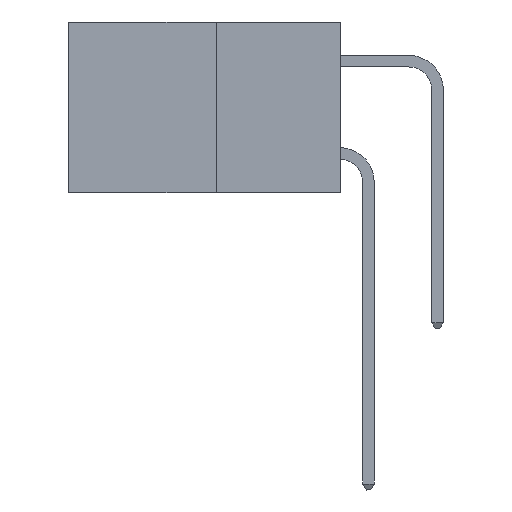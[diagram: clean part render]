
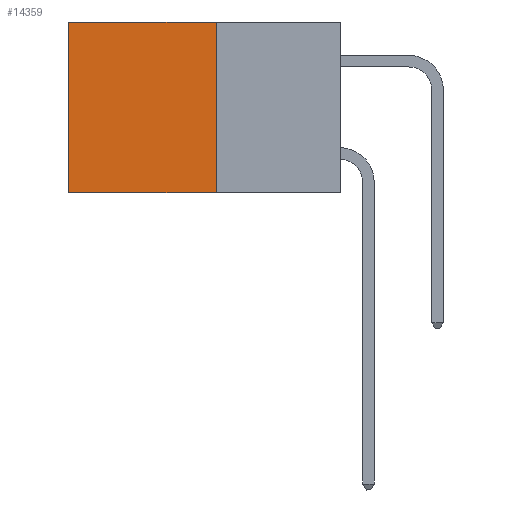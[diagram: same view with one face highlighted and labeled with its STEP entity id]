
A CAD part, left-side view. The second image highlights one B-rep face of the part: STEP entity #14359.
In plain terms, the highlighted planar face has unit normal (-1, 0, 0).
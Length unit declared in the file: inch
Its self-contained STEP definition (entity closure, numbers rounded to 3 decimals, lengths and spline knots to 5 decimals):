
#228 = VECTOR ( 'NONE', #15849, 39.37008 ) ;
#976 = DIRECTION ( 'NONE',  ( 0., 0., -1. ) ) ;
#2099 = VECTOR ( 'NONE', #976, 39.37008 ) ;
#2131 = FACE_OUTER_BOUND ( 'NONE', #4320, .T. ) ;
#3028 = VERTEX_POINT ( 'NONE', #15175 ) ;
#4080 = DIRECTION ( 'NONE',  ( 1., 0., 0. ) ) ;
#4320 = EDGE_LOOP ( 'NONE', ( #19175, #17777, #12674, #13110 ) ) ;
#4397 = CARTESIAN_POINT ( 'NONE',  ( 0.277, 0.59, -0.37 ) ) ;
#5639 = LINE ( 'NONE', #15153, #228 ) ;
#6575 = EDGE_CURVE ( 'NONE', #3028, #13908, #5639, .T. ) ;
#7083 = AXIS2_PLACEMENT_3D ( 'NONE', #14992, #4080, #16765 ) ;
#10024 = CARTESIAN_POINT ( 'NONE',  ( 0.277, 0.59, -0.37 ) ) ;
#10498 = DIRECTION ( 'NONE',  ( 0., 0., -1. ) ) ;
#11461 = CARTESIAN_POINT ( 'NONE',  ( 0.277, 0.27, 0. ) ) ;
#11939 = CARTESIAN_POINT ( 'NONE',  ( 0.277, 0.27, 0. ) ) ;
#12385 = LINE ( 'NONE', #10024, #2099 ) ;
#12674 = ORIENTED_EDGE ( 'NONE', *, *, #19387, .F. ) ;
#13110 = ORIENTED_EDGE ( 'NONE', *, *, #18531, .T. ) ;
#13908 = VERTEX_POINT ( 'NONE', #4397 ) ;
#14359 = ADVANCED_FACE ( 'NONE', ( #2131 ), #21924, .F. ) ;
#14992 = CARTESIAN_POINT ( 'NONE',  ( 0.277, 0.27, -0.37 ) ) ;
#15153 = CARTESIAN_POINT ( 'NONE',  ( 0.277, 0.27, -0.37 ) ) ;
#15175 = CARTESIAN_POINT ( 'NONE',  ( 0.277, 0.27, -0.37 ) ) ;
#15567 = DIRECTION ( 'NONE',  ( 0., 1., 0. ) ) ;
#15849 = DIRECTION ( 'NONE',  ( 0., 1., 0. ) ) ;
#16566 = CARTESIAN_POINT ( 'NONE',  ( 0.277, 0.59, 0. ) ) ;
#16646 = EDGE_CURVE ( 'NONE', #21040, #13908, #12385, .T. ) ;
#16765 = DIRECTION ( 'NONE',  ( 0., 0., -1. ) ) ;
#17548 = VECTOR ( 'NONE', #10498, 39.37008 ) ;
#17758 = VERTEX_POINT ( 'NONE', #11461 ) ;
#17777 = ORIENTED_EDGE ( 'NONE', *, *, #6575, .F. ) ;
#18391 = LINE ( 'NONE', #11939, #21903 ) ;
#18531 = EDGE_CURVE ( 'NONE', #17758, #21040, #18391, .T. ) ;
#19175 = ORIENTED_EDGE ( 'NONE', *, *, #16646, .T. ) ;
#19387 = EDGE_CURVE ( 'NONE', #17758, #3028, #22165, .T. ) ;
#19397 = CARTESIAN_POINT ( 'NONE',  ( 0.277, 0.27, -0.37 ) ) ;
#21040 = VERTEX_POINT ( 'NONE', #16566 ) ;
#21903 = VECTOR ( 'NONE', #15567, 39.37008 ) ;
#21924 = PLANE ( 'NONE',  #7083 ) ;
#22165 = LINE ( 'NONE', #19397, #17548 ) ;
